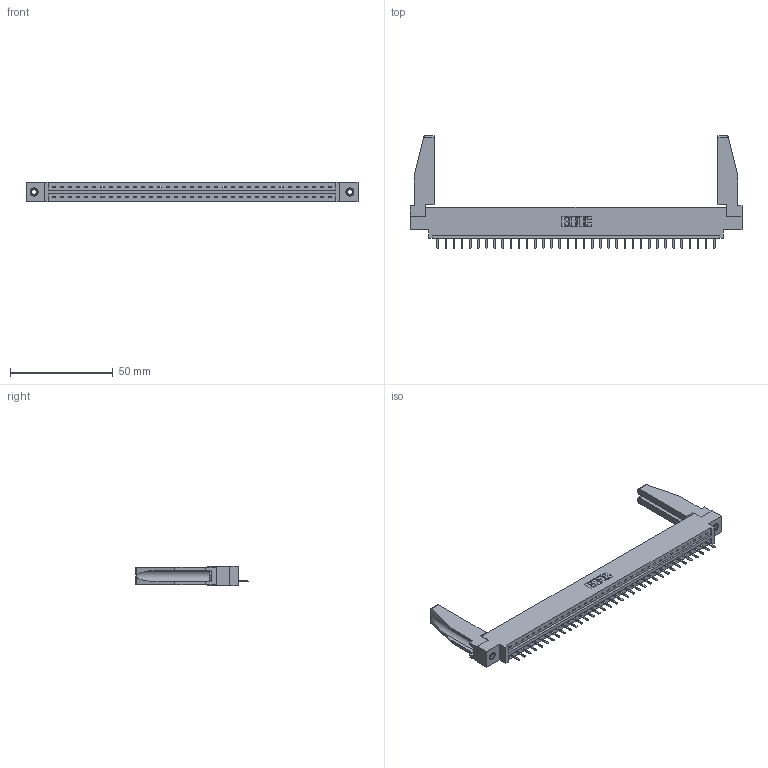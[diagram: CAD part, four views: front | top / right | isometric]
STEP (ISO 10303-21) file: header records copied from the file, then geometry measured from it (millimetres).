
FILE_DESCRIPTION (( 'STEP AP203' ), '1' );
FILE_NAME ('337-035-520-678.STEP', '2019-10-01T12:33:31', ( '' ), ( '' ), 'SwSTEP 2.0', 'SolidWorks 2016', '' );
FILE_SCHEMA (( 'CONFIG_CONTROL_DESIGN' ));
Length unit declared in the file: inch
Products named in the file (5): 337 Part_0.170 Offset - 0.156 Dia-TI; 337-035-520-678; 345-292-001_345-293-120; 345-250-001_345-250-001-102; 307-220-078
Assembly tree (40 placements, depth 2):
  337-035-520-678
    337 Part_0.170 Offset - 0.156 Dia-TI
    345-292-001_345-293-120  x35
    345-250-001_345-250-001-102  x2
    307-220-078  x2
Bounding box: 161.7 x 54.82 x 9.4 mm (x, y, z)
Volume: 20493.2 mm3; surface area: 20582.2 mm2
Topology: 40 solids, 40 shells, 2558 faces, 7513 edges, 4906 vertices
Faces by surface type: plane 1838, cylinder 704, cone 12, torus 4
Entity records: 29608 total; most frequent: CARTESIAN_POINT 5161, ORIENTED_EDGE 5076, DIRECTION 4356, EDGE_CURVE 2538, LINE 2368, VECTOR 2368, VERTEX_POINT 1684, AXIS2_PLACEMENT_3D 994
